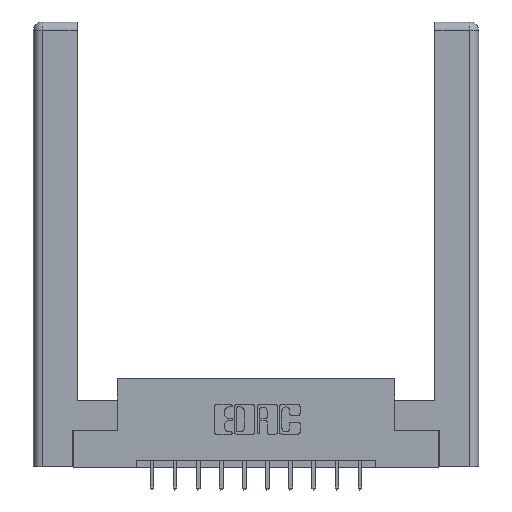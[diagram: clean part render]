
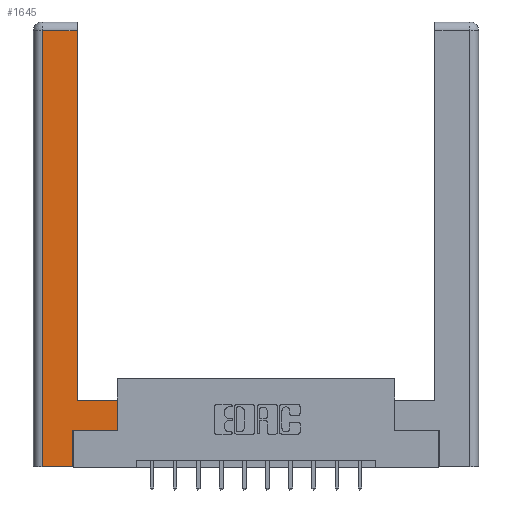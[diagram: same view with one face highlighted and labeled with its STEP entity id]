
A CAD part, top view. The second image highlights one B-rep face of the part: STEP entity #1645.
In plain terms, the highlighted planar face has unit normal (0, 0, 1).
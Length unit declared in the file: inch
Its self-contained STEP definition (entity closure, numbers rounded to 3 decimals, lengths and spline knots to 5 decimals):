
#259 = VERTEX_POINT ( 'NONE', #7732 ) ;
#857 = EDGE_CURVE ( 'NONE', #4764, #11452, #5227, .T. ) ;
#1029 = ORIENTED_EDGE ( 'NONE', *, *, #1865, .T. ) ;
#1571 = CARTESIAN_POINT ( 'NONE',  ( 0., 0., 0. ) ) ;
#1641 = LINE ( 'NONE', #10589, #10263 ) ;
#1645 = ADVANCED_FACE ( 'NONE', ( #6231 ), #8295, .F. ) ;
#1773 = VERTEX_POINT ( 'NONE', #3329 ) ;
#1865 = EDGE_CURVE ( 'NONE', #9456, #259, #9080, .T. ) ;
#2004 = ORIENTED_EDGE ( 'NONE', *, *, #10043, .T. ) ;
#2076 = CARTESIAN_POINT ( 'NONE',  ( 0.265, 0.245, 0. ) ) ;
#2092 = CARTESIAN_POINT ( 'NONE',  ( 0.295, 3., 0. ) ) ;
#2947 = CARTESIAN_POINT ( 'NONE',  ( 0.565, 0.45, 0. ) ) ;
#3329 = CARTESIAN_POINT ( 'NONE',  ( 0.295, 2.94, 0. ) ) ;
#3853 = DIRECTION ( 'NONE',  ( -1., 0., 0. ) ) ;
#4121 = ORIENTED_EDGE ( 'NONE', *, *, #8069, .T. ) ;
#4207 = LINE ( 'NONE', #9470, #6465 ) ;
#4217 = ORIENTED_EDGE ( 'NONE', *, *, #857, .T. ) ;
#4230 = EDGE_CURVE ( 'NONE', #14502, #9456, #6391, .T. ) ;
#4764 = VERTEX_POINT ( 'NONE', #2947 ) ;
#5227 = LINE ( 'NONE', #12969, #6780 ) ;
#5775 = VECTOR ( 'NONE', #13503, 39.37008 ) ;
#5886 = CARTESIAN_POINT ( 'NONE',  ( 0.0615, 0., 0. ) ) ;
#5977 = LINE ( 'NONE', #6539, #8956 ) ;
#6231 = FACE_OUTER_BOUND ( 'NONE', #7243, .T. ) ;
#6391 = LINE ( 'NONE', #5886, #13626 ) ;
#6415 = EDGE_CURVE ( 'NONE', #7052, #4764, #5977, .T. ) ;
#6434 = DIRECTION ( 'NONE',  ( -1., 0., 0. ) ) ;
#6465 = VECTOR ( 'NONE', #6434, 39.37008 ) ;
#6539 = CARTESIAN_POINT ( 'NONE',  ( 0.565, 0.45, 0. ) ) ;
#6570 = ORIENTED_EDGE ( 'NONE', *, *, #6415, .T. ) ;
#6780 = VECTOR ( 'NONE', #7361, 39.37008 ) ;
#6804 = DIRECTION ( 'NONE',  ( 1., 0., 0. ) ) ;
#7047 = VECTOR ( 'NONE', #11021, 39.37008 ) ;
#7052 = VERTEX_POINT ( 'NONE', #12655 ) ;
#7147 = LINE ( 'NONE', #9994, #5775 ) ;
#7243 = EDGE_LOOP ( 'NONE', ( #14321, #4121, #14395, #1029, #10472, #2004, #6570, #4217 ) ) ;
#7361 = DIRECTION ( 'NONE',  ( -1., 0., 0. ) ) ;
#7371 = CARTESIAN_POINT ( 'NONE',  ( 0.0615, 2.94, 0. ) ) ;
#7732 = CARTESIAN_POINT ( 'NONE',  ( 0.265, 0., 0. ) ) ;
#8069 = EDGE_CURVE ( 'NONE', #1773, #14502, #4207, .T. ) ;
#8295 = PLANE ( 'NONE',  #12054 ) ;
#8735 = CARTESIAN_POINT ( 'NONE',  ( 0.295, 0.45, 0. ) ) ;
#8956 = VECTOR ( 'NONE', #9937, 39.37008 ) ;
#9080 = LINE ( 'NONE', #11344, #9424 ) ;
#9424 = VECTOR ( 'NONE', #6804, 39.37008 ) ;
#9426 = DIRECTION ( 'NONE',  ( 0., 0., -1. ) ) ;
#9456 = VERTEX_POINT ( 'NONE', #9903 ) ;
#9470 = CARTESIAN_POINT ( 'NONE',  ( 0.0615, 2.94, 0. ) ) ;
#9514 = LINE ( 'NONE', #2092, #7047 ) ;
#9903 = CARTESIAN_POINT ( 'NONE',  ( 0.0615, 0., 0. ) ) ;
#9937 = DIRECTION ( 'NONE',  ( 0., 1., 0. ) ) ;
#9994 = CARTESIAN_POINT ( 'NONE',  ( 0.265, 0.245, 0. ) ) ;
#10043 = EDGE_CURVE ( 'NONE', #14280, #7052, #1641, .T. ) ;
#10263 = VECTOR ( 'NONE', #10643, 39.37008 ) ;
#10472 = ORIENTED_EDGE ( 'NONE', *, *, #14364, .T. ) ;
#10589 = CARTESIAN_POINT ( 'NONE',  ( 0.565, 0.245, 0. ) ) ;
#10643 = DIRECTION ( 'NONE',  ( 1., 0., 0. ) ) ;
#11021 = DIRECTION ( 'NONE',  ( 0., 1., 0. ) ) ;
#11344 = CARTESIAN_POINT ( 'NONE',  ( 0.265, 0., 0. ) ) ;
#11452 = VERTEX_POINT ( 'NONE', #8735 ) ;
#11841 = EDGE_CURVE ( 'NONE', #11452, #1773, #9514, .T. ) ;
#12054 = AXIS2_PLACEMENT_3D ( 'NONE', #1571, #9426, #3853 ) ;
#12655 = CARTESIAN_POINT ( 'NONE',  ( 0.565, 0.245, 0. ) ) ;
#12969 = CARTESIAN_POINT ( 'NONE',  ( 0.295, 0.45, 0. ) ) ;
#13503 = DIRECTION ( 'NONE',  ( 0., 1., 0. ) ) ;
#13626 = VECTOR ( 'NONE', #13747, 39.37008 ) ;
#13747 = DIRECTION ( 'NONE',  ( 0., -1., 0. ) ) ;
#14280 = VERTEX_POINT ( 'NONE', #2076 ) ;
#14321 = ORIENTED_EDGE ( 'NONE', *, *, #11841, .T. ) ;
#14364 = EDGE_CURVE ( 'NONE', #259, #14280, #7147, .T. ) ;
#14395 = ORIENTED_EDGE ( 'NONE', *, *, #4230, .T. ) ;
#14502 = VERTEX_POINT ( 'NONE', #7371 ) ;
